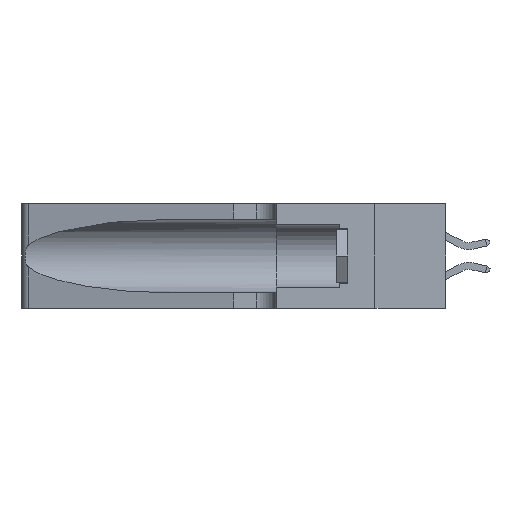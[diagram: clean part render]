
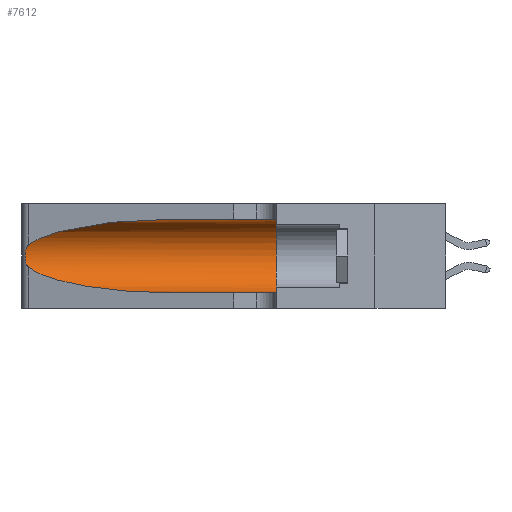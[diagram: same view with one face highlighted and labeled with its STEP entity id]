
A CAD part, left-side view. The second image highlights one B-rep face of the part: STEP entity #7612.
In plain terms, the highlighted cylindrical face has radius 3.308 mm (diameter 6.617 mm), a partial arc.
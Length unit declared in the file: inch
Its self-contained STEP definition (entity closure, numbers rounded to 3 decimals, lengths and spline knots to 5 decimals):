
#604 = EDGE_LOOP ( 'NONE', ( #18910, #27285, #26238, #30808, #10281, #18287 ) ) ;
#1422 = EDGE_CURVE ( 'NONE', #8124, #5703, #22356, .T. ) ;
#2616 = CARTESIAN_POINT ( 'NONE',  ( 0.25487, 1.22718, 0.22369 ) ) ;
#2769 = CARTESIAN_POINT ( 'NONE',  ( 0.25487, 1.22718, 0.14631 ) ) ;
#4159 = DIRECTION ( 'NONE',  ( 0., -1., 0. ) ) ;
#4261 = EDGE_CURVE ( 'NONE', #12910, #29404, #28796, .T. ) ;
#4454 = LINE ( 'NONE', #19322, #22230 ) ;
#4540 = VECTOR ( 'NONE', #20278, 39.37008 ) ;
#4634 = AXIS2_PLACEMENT_3D ( 'NONE', #26793, #21612, #28174 ) ;
#4990 = DIRECTION ( 'NONE',  ( 0., 0., -1. ) ) ;
#5395 = CARTESIAN_POINT ( 'NONE',  ( 0.25789, 1.23486, 0.15765 ) ) ;
#5703 = VERTEX_POINT ( 'NONE', #2616 ) ;
#6491 = CARTESIAN_POINT ( 'NONE',  ( 0.1305, 0.35, 0.05475 ) ) ;
#6993 = CARTESIAN_POINT ( 'NONE',  ( 0.26018, 1.23835, 0.19895 ) ) ;
#7070 = CARTESIAN_POINT ( 'NONE',  ( 0.1305, 1.61858, 0.185 ) ) ;
#7199 = CARTESIAN_POINT ( 'NONE',  ( 0.26017, 1.23833, 0.17102 ) ) ;
#7303 = CARTESIAN_POINT ( 'NONE',  ( 0.25787, 1.23484, 0.2124 ) ) ;
#7599 = CYLINDRICAL_SURFACE ( 'NONE', #13317, 0.13025 ) ;
#7612 = ADVANCED_FACE ( 'NONE', ( #13112 ), #7599, .F. ) ;
#8124 = VERTEX_POINT ( 'NONE', #28360 ) ;
#9100 = DIRECTION ( 'NONE',  ( 0., -1., 0. ) ) ;
#10281 = ORIENTED_EDGE ( 'NONE', *, *, #17426, .F. ) ;
#11872 = CARTESIAN_POINT ( 'NONE',  ( 0.25555, 1.22994, 0.2215 ) ) ;
#12197 = CARTESIAN_POINT ( 'NONE',  ( 0.26075, 1.23896, 0.178 ) ) ;
#12726 = CARTESIAN_POINT ( 'NONE',  ( 0.25555, 1.22993, 0.14849 ) ) ;
#12862 = EDGE_CURVE ( 'NONE', #29404, #15987, #4454, .T. ) ;
#12910 = VERTEX_POINT ( 'NONE', #19434 ) ;
#13112 = FACE_OUTER_BOUND ( 'NONE', #604, .T. ) ;
#13317 = AXIS2_PLACEMENT_3D ( 'NONE', #7070, #9100, #4990 ) ;
#13884 = EDGE_CURVE ( 'NONE', #5703, #12910, #16467, .T. ) ;
#14075 = CARTESIAN_POINT ( 'NONE',  ( 0.1305, 0.72297, 0.31525 ) ) ;
#14650 = CARTESIAN_POINT ( 'NONE',  ( 0.26075, 1.23896, 0.19203 ) ) ;
#14974 = CARTESIAN_POINT ( 'NONE',  ( 0.25854, 1.2359, 0.20912 ) ) ;
#15987 = VERTEX_POINT ( 'NONE', #6491 ) ;
#16365 = CARTESIAN_POINT ( 'NONE',  ( 0.18966, 0.96281, 0.31525 ) ) ;
#16467 = B_SPLINE_CURVE_WITH_KNOTS ( 'NONE', 3,
 ( #19181, #11872, #16974, #7303, #14974, #6993, #14650, #12197, #7199, #17905, #5395, #27836, #12726, #2769 ),
 .UNSPECIFIED., .F., .F.,
 ( 4, 2, 2, 2, 2, 2, 4 ),
 ( 0., 0.00027, 0.00053, 0.00107, 0.0016, 0.00187, 0.00214 ),
 .UNSPECIFIED. ) ;
#16974 = CARTESIAN_POINT ( 'NONE',  ( 0.25639, 1.23184, 0.21858 ) ) ;
#17426 = EDGE_CURVE ( 'NONE', #29719, #15987, #20777, .T. ) ;
#17905 = CARTESIAN_POINT ( 'NONE',  ( 0.25856, 1.23593, 0.16098 ) ) ;
#18287 = ORIENTED_EDGE ( 'NONE', *, *, #25997, .F. ) ;
#18910 = ORIENTED_EDGE ( 'NONE', *, *, #1422, .T. ) ;
#19052 = CARTESIAN_POINT ( 'NONE',  ( 0.25487, 1.22718, 0.22369 ) ) ;
#19181 = CARTESIAN_POINT ( 'NONE',  ( 0.25487, 1.22718, 0.22369 ) ) ;
#19322 = CARTESIAN_POINT ( 'NONE',  ( 0.1305, 1.61858, 0.05475 ) ) ;
#19434 = CARTESIAN_POINT ( 'NONE',  ( 0.25487, 1.22718, 0.14631 ) ) ;
#19575 = CARTESIAN_POINT ( 'NONE',  ( 0.25487, 1.22718, 0.14631 ) ) ;
#20132 = CARTESIAN_POINT ( 'NONE',  ( 0.1305, 0.35, 0.31525 ) ) ;
#20278 = DIRECTION ( 'NONE',  ( 0., -1., 0. ) ) ;
#20716 = LINE ( 'NONE', #25428, #4540 ) ;
#20777 = CIRCLE ( 'NONE', #4634, 0.13025 ) ;
#21612 = DIRECTION ( 'NONE',  ( 0., 1., 0. ) ) ;
#22230 = VECTOR ( 'NONE', #4159, 39.37008 ) ;
#22356 =( BOUNDED_CURVE ( )  B_SPLINE_CURVE ( 3, ( #14075, #16365, #23998, #19052 ),
 .UNSPECIFIED., .F., .F. ) 
 B_SPLINE_CURVE_WITH_KNOTS ( ( 4, 4 ),
 ( 1.5708, 2.84003 ),
 .UNSPECIFIED. ) 
 CURVE ( )  GEOMETRIC_REPRESENTATION_ITEM ( )  RATIONAL_B_SPLINE_CURVE ( ( 1., 0.87, 0.87, 1. ) ) 
 REPRESENTATION_ITEM ( '' )  );
#23998 = CARTESIAN_POINT ( 'NONE',  ( 0.2373, 1.15595, 0.28018 ) ) ;
#25428 = CARTESIAN_POINT ( 'NONE',  ( 0.1305, 1.61858, 0.31525 ) ) ;
#25997 = EDGE_CURVE ( 'NONE', #8124, #29719, #20716, .T. ) ;
#26238 = ORIENTED_EDGE ( 'NONE', *, *, #4261, .T. ) ;
#26247 = CARTESIAN_POINT ( 'NONE',  ( 0.1305, 0.72297, 0.05475 ) ) ;
#26793 = CARTESIAN_POINT ( 'NONE',  ( 0.1305, 0.35, 0.185 ) ) ;
#27285 = ORIENTED_EDGE ( 'NONE', *, *, #13884, .T. ) ;
#27836 = CARTESIAN_POINT ( 'NONE',  ( 0.25639, 1.23186, 0.15144 ) ) ;
#28117 = CARTESIAN_POINT ( 'NONE',  ( 0.18966, 0.96281, 0.05475 ) ) ;
#28174 = DIRECTION ( 'NONE',  ( 0., 0., 1. ) ) ;
#28360 = CARTESIAN_POINT ( 'NONE',  ( 0.1305, 0.72297, 0.31525 ) ) ;
#28796 =( BOUNDED_CURVE ( )  B_SPLINE_CURVE ( 3, ( #19575, #32624, #28117, #26247 ),
 .UNSPECIFIED., .F., .F. ) 
 B_SPLINE_CURVE_WITH_KNOTS ( ( 4, 4 ),
 ( 3.44316, 4.71239 ),
 .UNSPECIFIED. ) 
 CURVE ( )  GEOMETRIC_REPRESENTATION_ITEM ( )  RATIONAL_B_SPLINE_CURVE ( ( 1., 0.87, 0.87, 1. ) ) 
 REPRESENTATION_ITEM ( '' )  );
#28939 = CARTESIAN_POINT ( 'NONE',  ( 0.1305, 0.72297, 0.05475 ) ) ;
#29404 = VERTEX_POINT ( 'NONE', #28939 ) ;
#29719 = VERTEX_POINT ( 'NONE', #20132 ) ;
#30808 = ORIENTED_EDGE ( 'NONE', *, *, #12862, .T. ) ;
#32624 = CARTESIAN_POINT ( 'NONE',  ( 0.2373, 1.15595, 0.08982 ) ) ;
